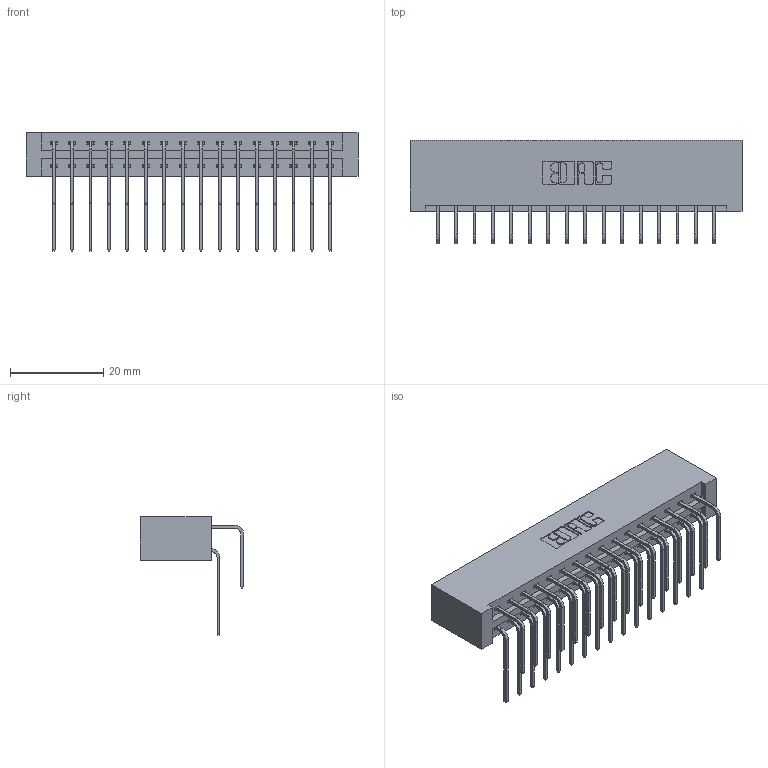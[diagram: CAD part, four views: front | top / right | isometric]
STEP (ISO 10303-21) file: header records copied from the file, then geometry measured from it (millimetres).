
FILE_DESCRIPTION (( 'STEP AP203' ), '1' );
FILE_NAME ('387-032-558-201.STEP', '2018-09-18T08:11:31', ( '' ), ( '' ), 'SwSTEP 2.0', 'SolidWorks 2016', '' );
FILE_SCHEMA (( 'CONFIG_CONTROL_DESIGN' ));
Length unit declared in the file: inch
Products named in the file (4): 337 Part_No Mounting Lugs; 345-292-001_558 559 Tail - 1; 345-292-001_558 Tail - 2; 387-032-558-201
Assembly tree (33 placements, depth 2):
  387-032-558-201
    337 Part_No Mounting Lugs
    345-292-001_558 559 Tail - 1  x16
    345-292-001_558 Tail - 2  x16
Bounding box: 71.27 x 22.17 x 25.53 mm (x, y, z)
Volume: 8110.5 mm3; surface area: 9899.4 mm2
Topology: 33 solids, 33 shells, 1898 faces, 5631 edges, 3710 vertices
Faces by surface type: plane 1346, cylinder 552
Entity records: 17275 total; most frequent: CARTESIAN_POINT 2977, ORIENTED_EDGE 2862, DIRECTION 2555, EDGE_CURVE 1431, VECTOR 1271, LINE 1271, VERTEX_POINT 950, AXIS2_PLACEMENT_3D 642
